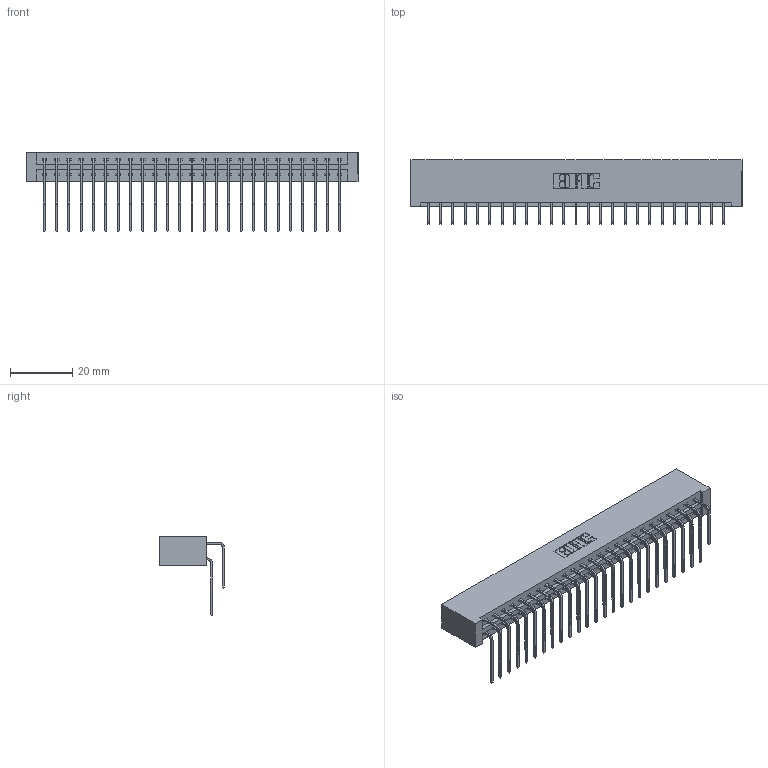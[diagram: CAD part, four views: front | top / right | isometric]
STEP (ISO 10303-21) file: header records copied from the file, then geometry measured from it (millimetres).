
FILE_DESCRIPTION (( 'STEP AP203' ), '1' );
FILE_NAME ('387-050-559-201.STEP', '2018-09-20T09:13:03', ( '' ), ( '' ), 'SwSTEP 2.0', 'SolidWorks 2016', '' );
FILE_SCHEMA (( 'CONFIG_CONTROL_DESIGN' ));
Length unit declared in the file: inch
Products named in the file (4): 337 Part_No Mounting Lugs; 345-292-001_558 559 Tail - 1; 345-292-001_559 Tail - 2; 387-050-559-201
Assembly tree (51 placements, depth 2):
  387-050-559-201
    337 Part_No Mounting Lugs
    345-292-001_558 559 Tail - 1  x25
    345-292-001_559 Tail - 2  x25
Bounding box: 106.93 x 20.9 x 25.53 mm (x, y, z)
Volume: 12092.4 mm3; surface area: 15009.8 mm2
Topology: 51 solids, 51 shells, 2906 faces, 8637 edges, 5690 vertices
Faces by surface type: plane 2066, cylinder 840
Entity records: 23089 total; most frequent: CARTESIAN_POINT 3949, ORIENTED_EDGE 3834, DIRECTION 3365, EDGE_CURVE 1917, LINE 1757, VECTOR 1757, VERTEX_POINT 1274, AXIS2_PLACEMENT_3D 804
